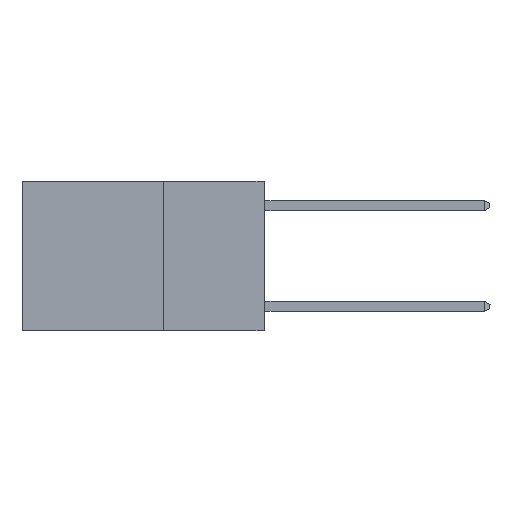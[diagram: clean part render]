
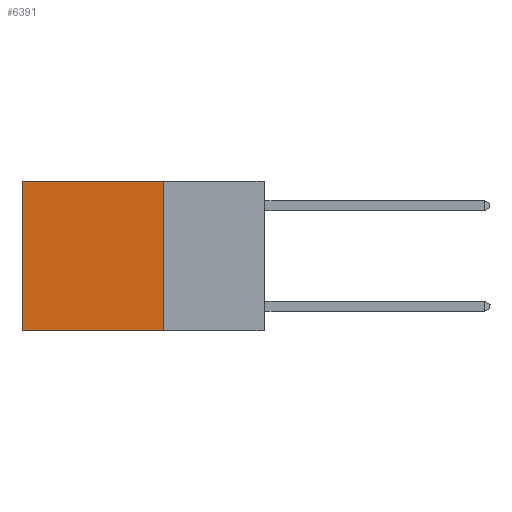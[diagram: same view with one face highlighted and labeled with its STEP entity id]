
A CAD part, left-side view. The second image highlights one B-rep face of the part: STEP entity #6391.
In plain terms, the highlighted planar face has unit normal (-1, 0, 0).
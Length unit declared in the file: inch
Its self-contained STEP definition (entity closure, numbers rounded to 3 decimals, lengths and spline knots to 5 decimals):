
#72 = EDGE_CURVE ( 'NONE', #16689, #4703, #18075, .T. ) ;
#474 = DIRECTION ( 'NONE',  ( 0., 1., 0. ) ) ;
#1648 = DIRECTION ( 'NONE',  ( 0., 0., -1. ) ) ;
#2384 = DIRECTION ( 'NONE',  ( 0., 1., 0. ) ) ;
#3275 = VECTOR ( 'NONE', #28705, 39.37008 ) ;
#4703 = VERTEX_POINT ( 'NONE', #23771 ) ;
#6281 = VECTOR ( 'NONE', #8225, 39.37008 ) ;
#6391 = ADVANCED_FACE ( 'NONE', ( #30485 ), #28611, .F. ) ;
#6651 = CARTESIAN_POINT ( 'NONE',  ( 0.2625, 0.25, 0. ) ) ;
#7064 = LINE ( 'NONE', #15582, #6281 ) ;
#7290 = CARTESIAN_POINT ( 'NONE',  ( 0.2625, 0.25, -0.37 ) ) ;
#8225 = DIRECTION ( 'NONE',  ( 0., 0., -1. ) ) ;
#9919 = LINE ( 'NONE', #6651, #3275 ) ;
#10601 = ORIENTED_EDGE ( 'NONE', *, *, #13708, .F. ) ;
#13372 = EDGE_LOOP ( 'NONE', ( #26223, #10601, #18608, #30925 ) ) ;
#13708 = EDGE_CURVE ( 'NONE', #28588, #15939, #25463, .T. ) ;
#13782 = CARTESIAN_POINT ( 'NONE',  ( 0.2625, 0.25, 0. ) ) ;
#14052 = CARTESIAN_POINT ( 'NONE',  ( 0.2625, 0.25, 0. ) ) ;
#15582 = CARTESIAN_POINT ( 'NONE',  ( 0.2625, 0.6, 0. ) ) ;
#15939 = VERTEX_POINT ( 'NONE', #16072 ) ;
#16072 = CARTESIAN_POINT ( 'NONE',  ( 0.2625, 0.6, -0.37 ) ) ;
#16504 = DIRECTION ( 'NONE',  ( 1., 0., 0. ) ) ;
#16689 = VERTEX_POINT ( 'NONE', #13782 ) ;
#17485 = CARTESIAN_POINT ( 'NONE',  ( 0.2625, 0.25, -0.37 ) ) ;
#18075 = LINE ( 'NONE', #29891, #30201 ) ;
#18608 = ORIENTED_EDGE ( 'NONE', *, *, #25039, .F. ) ;
#18996 = VECTOR ( 'NONE', #2384, 39.37008 ) ;
#20094 = EDGE_CURVE ( 'NONE', #4703, #15939, #7064, .T. ) ;
#23771 = CARTESIAN_POINT ( 'NONE',  ( 0.2625, 0.6, 0. ) ) ;
#25039 = EDGE_CURVE ( 'NONE', #16689, #28588, #9919, .T. ) ;
#25463 = LINE ( 'NONE', #7290, #18996 ) ;
#26223 = ORIENTED_EDGE ( 'NONE', *, *, #20094, .T. ) ;
#28588 = VERTEX_POINT ( 'NONE', #17485 ) ;
#28611 = PLANE ( 'NONE',  #30730 ) ;
#28705 = DIRECTION ( 'NONE',  ( 0., 0., -1. ) ) ;
#29891 = CARTESIAN_POINT ( 'NONE',  ( 0.2625, 0.25, 0. ) ) ;
#30201 = VECTOR ( 'NONE', #474, 39.37008 ) ;
#30485 = FACE_OUTER_BOUND ( 'NONE', #13372, .T. ) ;
#30730 = AXIS2_PLACEMENT_3D ( 'NONE', #14052, #16504, #1648 ) ;
#30925 = ORIENTED_EDGE ( 'NONE', *, *, #72, .T. ) ;
